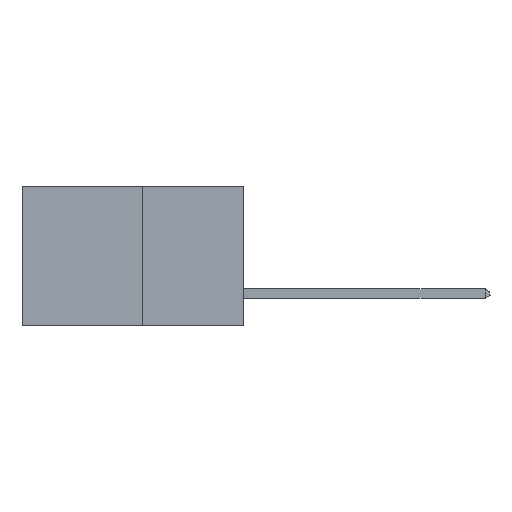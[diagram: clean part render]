
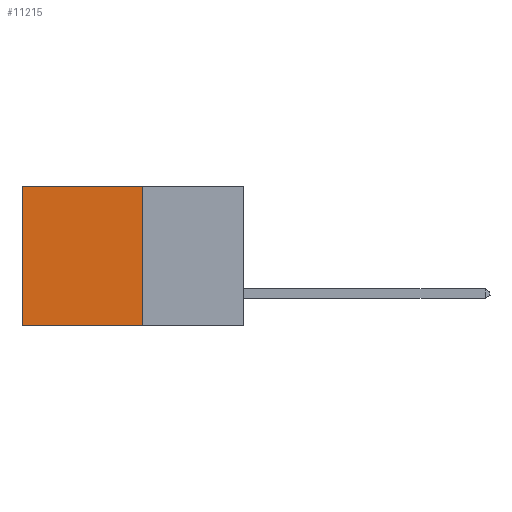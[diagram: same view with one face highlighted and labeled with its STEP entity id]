
A CAD part, left-side view. The second image highlights one B-rep face of the part: STEP entity #11215.
In plain terms, the highlighted planar face has unit normal (-1, 0, 0).
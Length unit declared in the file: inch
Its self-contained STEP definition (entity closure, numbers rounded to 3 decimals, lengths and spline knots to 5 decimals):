
#168 = EDGE_CURVE ( 'NONE', #1325, #9657, #25510, .T. ) ;
#382 = VECTOR ( 'NONE', #1541, 39.37008 ) ;
#456 = CARTESIAN_POINT ( 'NONE',  ( 0.277, 0.27, -0.37 ) ) ;
#1171 = LINE ( 'NONE', #26060, #382 ) ;
#1325 = VERTEX_POINT ( 'NONE', #14098 ) ;
#1541 = DIRECTION ( 'NONE',  ( 0., 0., -1. ) ) ;
#2188 = FACE_OUTER_BOUND ( 'NONE', #4232, .T. ) ;
#4232 = EDGE_LOOP ( 'NONE', ( #10250, #18185, #5136, #29964 ) ) ;
#5001 = DIRECTION ( 'NONE',  ( 0., 1., 0. ) ) ;
#5136 = ORIENTED_EDGE ( 'NONE', *, *, #28158, .F. ) ;
#6233 = CARTESIAN_POINT ( 'NONE',  ( 0.277, 0.27, -0.37 ) ) ;
#6911 = EDGE_CURVE ( 'NONE', #13345, #31102, #11096, .T. ) ;
#7408 = CARTESIAN_POINT ( 'NONE',  ( 0.277, 0.27, -0.37 ) ) ;
#8479 = LINE ( 'NONE', #6233, #21094 ) ;
#8743 = DIRECTION ( 'NONE',  ( 0., 0., -1. ) ) ;
#9657 = VERTEX_POINT ( 'NONE', #26093 ) ;
#10250 = ORIENTED_EDGE ( 'NONE', *, *, #25481, .T. ) ;
#11096 = LINE ( 'NONE', #7408, #31115 ) ;
#11215 = ADVANCED_FACE ( 'NONE', ( #2188 ), #24708, .F. ) ;
#13345 = VERTEX_POINT ( 'NONE', #456 ) ;
#14098 = CARTESIAN_POINT ( 'NONE',  ( 0.277, 0.27, 0. ) ) ;
#18185 = ORIENTED_EDGE ( 'NONE', *, *, #6911, .F. ) ;
#18617 = CARTESIAN_POINT ( 'NONE',  ( 0.277, 0.59, -0.37 ) ) ;
#19524 = DIRECTION ( 'NONE',  ( 0., 0., -1. ) ) ;
#21094 = VECTOR ( 'NONE', #8743, 39.37008 ) ;
#22100 = CARTESIAN_POINT ( 'NONE',  ( 0.277, 0.27, 0. ) ) ;
#22572 = DIRECTION ( 'NONE',  ( 0., 1., 0. ) ) ;
#24708 = PLANE ( 'NONE',  #26836 ) ;
#25481 = EDGE_CURVE ( 'NONE', #9657, #31102, #1171, .T. ) ;
#25510 = LINE ( 'NONE', #22100, #32136 ) ;
#26060 = CARTESIAN_POINT ( 'NONE',  ( 0.277, 0.59, -0.37 ) ) ;
#26093 = CARTESIAN_POINT ( 'NONE',  ( 0.277, 0.59, 0. ) ) ;
#26836 = AXIS2_PLACEMENT_3D ( 'NONE', #32112, #27176, #19524 ) ;
#27176 = DIRECTION ( 'NONE',  ( 1., 0., 0. ) ) ;
#28158 = EDGE_CURVE ( 'NONE', #1325, #13345, #8479, .T. ) ;
#29964 = ORIENTED_EDGE ( 'NONE', *, *, #168, .T. ) ;
#31102 = VERTEX_POINT ( 'NONE', #18617 ) ;
#31115 = VECTOR ( 'NONE', #5001, 39.37008 ) ;
#32112 = CARTESIAN_POINT ( 'NONE',  ( 0.277, 0.27, -0.37 ) ) ;
#32136 = VECTOR ( 'NONE', #22572, 39.37008 ) ;
